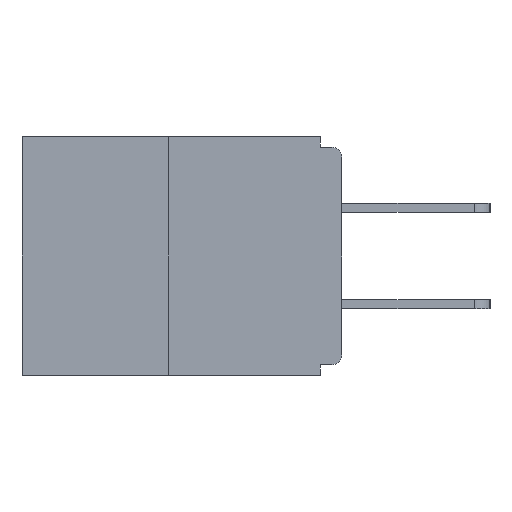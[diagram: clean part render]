
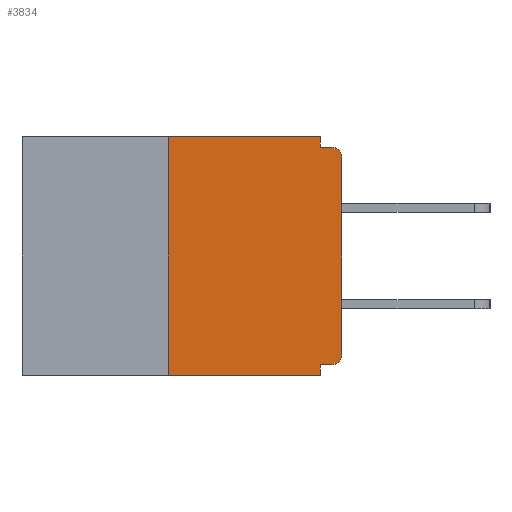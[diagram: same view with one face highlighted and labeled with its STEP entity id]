
A CAD part, left-side view. The second image highlights one B-rep face of the part: STEP entity #3834.
In plain terms, the highlighted planar face has unit normal (-1, 0, 0).
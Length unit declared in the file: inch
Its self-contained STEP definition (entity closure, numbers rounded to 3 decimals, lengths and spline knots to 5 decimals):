
#79 = VECTOR ( 'NONE', #519, 39.37008 ) ;
#519 = DIRECTION ( 'NONE',  ( 0., 0., -1. ) ) ;
#806 = DIRECTION ( 'NONE',  ( 0., 0., 1. ) ) ;
#889 = EDGE_CURVE ( 'NONE', #12667, #10250, #5177, .T. ) ;
#1083 = DIRECTION ( 'NONE',  ( 0., 1., 0. ) ) ;
#1250 = CARTESIAN_POINT ( 'NONE',  ( 0., 0.25, -0.343 ) ) ;
#1299 = VECTOR ( 'NONE', #3093, 39.37008 ) ;
#1569 = CARTESIAN_POINT ( 'NONE',  ( 0., 0.031, 0. ) ) ;
#2060 = CARTESIAN_POINT ( 'NONE',  ( 0., 0.015, -0.015 ) ) ;
#2175 = EDGE_CURVE ( 'NONE', #10250, #5551, #13553, .T. ) ;
#2236 = ORIENTED_EDGE ( 'NONE', *, *, #889, .F. ) ;
#2345 = DIRECTION ( 'NONE',  ( 1., 0., 0. ) ) ;
#2406 = VERTEX_POINT ( 'NONE', #7879 ) ;
#2481 = CARTESIAN_POINT ( 'NONE',  ( 0., 0.46, -0.343 ) ) ;
#2753 = ORIENTED_EDGE ( 'NONE', *, *, #2175, .F. ) ;
#2860 = AXIS2_PLACEMENT_3D ( 'NONE', #10216, #12888, #9276 ) ;
#3093 = DIRECTION ( 'NONE',  ( 0., 0., -1. ) ) ;
#3156 = VECTOR ( 'NONE', #10983, 39.37008 ) ;
#3455 = EDGE_CURVE ( 'NONE', #2406, #4928, #3957, .T. ) ;
#3834 = ADVANCED_FACE ( 'NONE', ( #3866 ), #15356, .F. ) ;
#3866 = FACE_OUTER_BOUND ( 'NONE', #11244, .T. ) ;
#3957 = CIRCLE ( 'NONE', #2860, 0.015 ) ;
#4421 = VECTOR ( 'NONE', #4701, 39.37008 ) ;
#4584 = CARTESIAN_POINT ( 'NONE',  ( 0., 0.25, 0. ) ) ;
#4668 = EDGE_CURVE ( 'NONE', #8032, #12779, #4893, .T. ) ;
#4701 = DIRECTION ( 'NONE',  ( 0., -1., 0. ) ) ;
#4893 = LINE ( 'NONE', #7559, #12697 ) ;
#4928 = VERTEX_POINT ( 'NONE', #2060 ) ;
#5177 = LINE ( 'NONE', #12818, #5767 ) ;
#5186 = EDGE_CURVE ( 'NONE', #12667, #14829, #16757, .T. ) ;
#5245 = DIRECTION ( 'NONE',  ( 0., 0., 1. ) ) ;
#5551 = VERTEX_POINT ( 'NONE', #15377 ) ;
#5556 = CARTESIAN_POINT ( 'NONE',  ( 0., 0.031, -0.328 ) ) ;
#5575 = CARTESIAN_POINT ( 'NONE',  ( 0., 0.031, 0. ) ) ;
#5696 = ORIENTED_EDGE ( 'NONE', *, *, #13668, .T. ) ;
#5704 = EDGE_CURVE ( 'NONE', #12779, #7950, #9776, .T. ) ;
#5767 = VECTOR ( 'NONE', #1083, 39.37008 ) ;
#7192 = ORIENTED_EDGE ( 'NONE', *, *, #4668, .F. ) ;
#7430 = ORIENTED_EDGE ( 'NONE', *, *, #5186, .T. ) ;
#7559 = CARTESIAN_POINT ( 'NONE',  ( 0., 0.46, 0. ) ) ;
#7658 = EDGE_CURVE ( 'NONE', #7950, #4928, #16464, .T. ) ;
#7879 = CARTESIAN_POINT ( 'NONE',  ( 0., 0., -0.03 ) ) ;
#7950 = VERTEX_POINT ( 'NONE', #16031 ) ;
#8032 = VERTEX_POINT ( 'NONE', #8130 ) ;
#8130 = CARTESIAN_POINT ( 'NONE',  ( 0., 0.25, 0. ) ) ;
#8755 = CARTESIAN_POINT ( 'NONE',  ( 0., 0., -0.313 ) ) ;
#9182 = LINE ( 'NONE', #15980, #9410 ) ;
#9276 = DIRECTION ( 'NONE',  ( 0., 0., -1. ) ) ;
#9347 = AXIS2_PLACEMENT_3D ( 'NONE', #15844, #15924, #14539 ) ;
#9410 = VECTOR ( 'NONE', #5245, 39.37008 ) ;
#9547 = ORIENTED_EDGE ( 'NONE', *, *, #15886, .F. ) ;
#9776 = LINE ( 'NONE', #5575, #79 ) ;
#10216 = CARTESIAN_POINT ( 'NONE',  ( 0., 0.015, -0.03 ) ) ;
#10250 = VERTEX_POINT ( 'NONE', #5556 ) ;
#10601 = VERTEX_POINT ( 'NONE', #1250 ) ;
#10983 = DIRECTION ( 'NONE',  ( 0., -1., 0. ) ) ;
#11086 = LINE ( 'NONE', #4584, #13010 ) ;
#11244 = EDGE_LOOP ( 'NONE', ( #7192, #9547, #12260, #2753, #2236, #7430, #5696, #14916, #16809, #15570 ) ) ;
#11275 = EDGE_CURVE ( 'NONE', #10601, #5551, #15100, .T. ) ;
#11459 = CARTESIAN_POINT ( 'NONE',  ( 0., 0., -0.015 ) ) ;
#12260 = ORIENTED_EDGE ( 'NONE', *, *, #11275, .T. ) ;
#12667 = VERTEX_POINT ( 'NONE', #14423 ) ;
#12697 = VECTOR ( 'NONE', #16817, 39.37008 ) ;
#12779 = VERTEX_POINT ( 'NONE', #1569 ) ;
#12818 = CARTESIAN_POINT ( 'NONE',  ( 0., 0., -0.328 ) ) ;
#12888 = DIRECTION ( 'NONE',  ( -1., 0., 0. ) ) ;
#13010 = VECTOR ( 'NONE', #806, 39.37008 ) ;
#13553 = LINE ( 'NONE', #14830, #1299 ) ;
#13668 = EDGE_CURVE ( 'NONE', #14829, #2406, #9182, .T. ) ;
#13903 = AXIS2_PLACEMENT_3D ( 'NONE', #16962, #2345, #14173 ) ;
#14173 = DIRECTION ( 'NONE',  ( 0., 0., -1. ) ) ;
#14423 = CARTESIAN_POINT ( 'NONE',  ( 0., 0.015, -0.328 ) ) ;
#14539 = DIRECTION ( 'NONE',  ( 0., 0., -1. ) ) ;
#14829 = VERTEX_POINT ( 'NONE', #8755 ) ;
#14830 = CARTESIAN_POINT ( 'NONE',  ( 0., 0.031, -0.343 ) ) ;
#14916 = ORIENTED_EDGE ( 'NONE', *, *, #3455, .T. ) ;
#15100 = LINE ( 'NONE', #2481, #3156 ) ;
#15356 = PLANE ( 'NONE',  #13903 ) ;
#15377 = CARTESIAN_POINT ( 'NONE',  ( 0., 0.031, -0.343 ) ) ;
#15570 = ORIENTED_EDGE ( 'NONE', *, *, #5704, .F. ) ;
#15844 = CARTESIAN_POINT ( 'NONE',  ( 0., 0.015, -0.313 ) ) ;
#15886 = EDGE_CURVE ( 'NONE', #10601, #8032, #11086, .T. ) ;
#15924 = DIRECTION ( 'NONE',  ( -1., 0., 0. ) ) ;
#15980 = CARTESIAN_POINT ( 'NONE',  ( 0., 0., 0. ) ) ;
#16031 = CARTESIAN_POINT ( 'NONE',  ( 0., 0.031, -0.015 ) ) ;
#16464 = LINE ( 'NONE', #11459, #4421 ) ;
#16757 = CIRCLE ( 'NONE', #9347, 0.015 ) ;
#16809 = ORIENTED_EDGE ( 'NONE', *, *, #7658, .F. ) ;
#16817 = DIRECTION ( 'NONE',  ( 0., -1., 0. ) ) ;
#16962 = CARTESIAN_POINT ( 'NONE',  ( 0., 0.46, 0. ) ) ;
